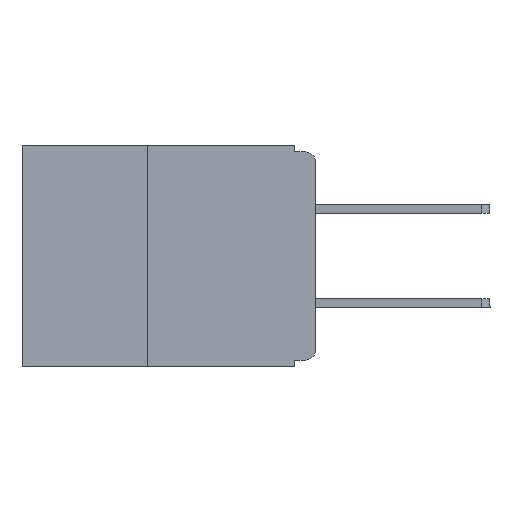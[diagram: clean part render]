
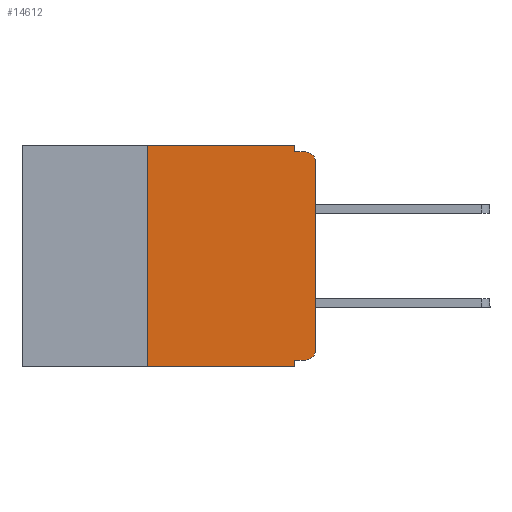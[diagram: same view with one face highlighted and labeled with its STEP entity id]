
A CAD part, left-side view. The second image highlights one B-rep face of the part: STEP entity #14612.
In plain terms, the highlighted planar face has unit normal (-1, 0, 0).
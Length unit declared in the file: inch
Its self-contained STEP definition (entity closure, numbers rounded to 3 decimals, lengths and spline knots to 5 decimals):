
#146 = VERTEX_POINT ( 'NONE', #7642 ) ;
#563 = CARTESIAN_POINT ( 'NONE',  ( 0., 0., -0.305 ) ) ;
#1177 = VERTEX_POINT ( 'NONE', #3852 ) ;
#1199 = DIRECTION ( 'NONE',  ( 0., 0., -1. ) ) ;
#1212 = CARTESIAN_POINT ( 'NONE',  ( 0., 0., -0.025 ) ) ;
#1380 = DIRECTION ( 'NONE',  ( 0., 0., -1. ) ) ;
#1397 = DIRECTION ( 'NONE',  ( 0., 0., -1. ) ) ;
#1670 = ORIENTED_EDGE ( 'NONE', *, *, #18546, .T. ) ;
#2385 = LINE ( 'NONE', #8615, #6487 ) ;
#2807 = LINE ( 'NONE', #14446, #3311 ) ;
#3034 = VERTEX_POINT ( 'NONE', #1212 ) ;
#3311 = VECTOR ( 'NONE', #6911, 39.37008 ) ;
#3441 = EDGE_CURVE ( 'NONE', #15234, #1177, #16899, .T. ) ;
#3852 = CARTESIAN_POINT ( 'NONE',  ( 0., 0.015, -0.01 ) ) ;
#3988 = DIRECTION ( 'NONE',  ( 0., 1., 0. ) ) ;
#4159 = LINE ( 'NONE', #13452, #8696 ) ;
#4619 = CARTESIAN_POINT ( 'NONE',  ( 0., 0.015, -0.32 ) ) ;
#4626 = ORIENTED_EDGE ( 'NONE', *, *, #19407, .T. ) ;
#5005 = ORIENTED_EDGE ( 'NONE', *, *, #7294, .F. ) ;
#5114 = VERTEX_POINT ( 'NONE', #18525 ) ;
#5192 = CARTESIAN_POINT ( 'NONE',  ( 0., 0.437, -0.33 ) ) ;
#5337 = EDGE_CURVE ( 'NONE', #12491, #3034, #2385, .T. ) ;
#5947 = EDGE_LOOP ( 'NONE', ( #17070, #1670, #9372, #13876, #10310, #11251, #4626, #16771, #5005, #14297 ) ) ;
#6035 = AXIS2_PLACEMENT_3D ( 'NONE', #19416, #10554, #1380 ) ;
#6081 = EDGE_CURVE ( 'NONE', #10206, #146, #12570, .T. ) ;
#6108 = CARTESIAN_POINT ( 'NONE',  ( 0., 0.031, 0. ) ) ;
#6487 = VECTOR ( 'NONE', #13597, 39.37008 ) ;
#6739 = DIRECTION ( 'NONE',  ( 0., -1., 0. ) ) ;
#6911 = DIRECTION ( 'NONE',  ( 0., 0., -1. ) ) ;
#7294 = EDGE_CURVE ( 'NONE', #14668, #5114, #14885, .T. ) ;
#7605 = DIRECTION ( 'NONE',  ( 0., 0., -1. ) ) ;
#7619 = VECTOR ( 'NONE', #7605, 39.37008 ) ;
#7642 = CARTESIAN_POINT ( 'NONE',  ( 0., 0.25, 0. ) ) ;
#8070 = EDGE_CURVE ( 'NONE', #146, #11073, #4159, .T. ) ;
#8434 = VECTOR ( 'NONE', #11570, 39.37008 ) ;
#8492 = CIRCLE ( 'NONE', #6035, 0.015 ) ;
#8615 = CARTESIAN_POINT ( 'NONE',  ( 0., 0., 0. ) ) ;
#8696 = VECTOR ( 'NONE', #14975, 39.37008 ) ;
#9372 = ORIENTED_EDGE ( 'NONE', *, *, #3441, .F. ) ;
#10206 = VERTEX_POINT ( 'NONE', #10478 ) ;
#10310 = ORIENTED_EDGE ( 'NONE', *, *, #8070, .F. ) ;
#10371 = DIRECTION ( 'NONE',  ( -1., 0., 0. ) ) ;
#10478 = CARTESIAN_POINT ( 'NONE',  ( 0., 0.25, -0.33 ) ) ;
#10554 = DIRECTION ( 'NONE',  ( -1., 0., 0. ) ) ;
#10572 = DIRECTION ( 'NONE',  ( 1., 0., 0. ) ) ;
#10699 = CARTESIAN_POINT ( 'NONE',  ( 0., 0.25, -0.33 ) ) ;
#10782 = CIRCLE ( 'NONE', #12049, 0.015 ) ;
#10839 = DIRECTION ( 'NONE',  ( 0., 0., 1. ) ) ;
#11073 = VERTEX_POINT ( 'NONE', #14117 ) ;
#11251 = ORIENTED_EDGE ( 'NONE', *, *, #6081, .F. ) ;
#11570 = DIRECTION ( 'NONE',  ( 0., -1., 0. ) ) ;
#11604 = VECTOR ( 'NONE', #10839, 39.37008 ) ;
#11940 = VERTEX_POINT ( 'NONE', #17763 ) ;
#12013 = CARTESIAN_POINT ( 'NONE',  ( 0., 0.031, -0.01 ) ) ;
#12049 = AXIS2_PLACEMENT_3D ( 'NONE', #19240, #10371, #1199 ) ;
#12491 = VERTEX_POINT ( 'NONE', #563 ) ;
#12530 = EDGE_CURVE ( 'NONE', #5114, #11940, #2807, .T. ) ;
#12570 = LINE ( 'NONE', #10699, #11604 ) ;
#13103 = CARTESIAN_POINT ( 'NONE',  ( 0., 0., -0.32 ) ) ;
#13204 = CARTESIAN_POINT ( 'NONE',  ( 0., 0., -0.01 ) ) ;
#13330 = EDGE_CURVE ( 'NONE', #14668, #12491, #8492, .T. ) ;
#13422 = FACE_OUTER_BOUND ( 'NONE', #5947, .T. ) ;
#13452 = CARTESIAN_POINT ( 'NONE',  ( 0., 0.437, 0. ) ) ;
#13456 = VECTOR ( 'NONE', #3988, 39.37008 ) ;
#13597 = DIRECTION ( 'NONE',  ( 0., 0., 1. ) ) ;
#13876 = ORIENTED_EDGE ( 'NONE', *, *, #17031, .F. ) ;
#14117 = CARTESIAN_POINT ( 'NONE',  ( 0., 0.031, 0. ) ) ;
#14297 = ORIENTED_EDGE ( 'NONE', *, *, #13330, .T. ) ;
#14446 = CARTESIAN_POINT ( 'NONE',  ( 0., 0.031, -0.33 ) ) ;
#14612 = ADVANCED_FACE ( 'NONE', ( #13422 ), #19437, .F. ) ;
#14668 = VERTEX_POINT ( 'NONE', #4619 ) ;
#14885 = LINE ( 'NONE', #13103, #13456 ) ;
#14975 = DIRECTION ( 'NONE',  ( 0., -1., 0. ) ) ;
#15038 = VECTOR ( 'NONE', #6739, 39.37008 ) ;
#15087 = CARTESIAN_POINT ( 'NONE',  ( 0., 0.437, 0. ) ) ;
#15234 = VERTEX_POINT ( 'NONE', #12013 ) ;
#16771 = ORIENTED_EDGE ( 'NONE', *, *, #12530, .F. ) ;
#16899 = LINE ( 'NONE', #13204, #8434 ) ;
#17031 = EDGE_CURVE ( 'NONE', #11073, #15234, #19484, .T. ) ;
#17070 = ORIENTED_EDGE ( 'NONE', *, *, #5337, .T. ) ;
#17582 = AXIS2_PLACEMENT_3D ( 'NONE', #15087, #10572, #1397 ) ;
#17763 = CARTESIAN_POINT ( 'NONE',  ( 0., 0.031, -0.33 ) ) ;
#18427 = LINE ( 'NONE', #5192, #15038 ) ;
#18525 = CARTESIAN_POINT ( 'NONE',  ( 0., 0.031, -0.32 ) ) ;
#18546 = EDGE_CURVE ( 'NONE', #3034, #1177, #10782, .T. ) ;
#19240 = CARTESIAN_POINT ( 'NONE',  ( 0., 0.015, -0.025 ) ) ;
#19407 = EDGE_CURVE ( 'NONE', #10206, #11940, #18427, .T. ) ;
#19416 = CARTESIAN_POINT ( 'NONE',  ( 0., 0.015, -0.305 ) ) ;
#19437 = PLANE ( 'NONE',  #17582 ) ;
#19484 = LINE ( 'NONE', #6108, #7619 ) ;
